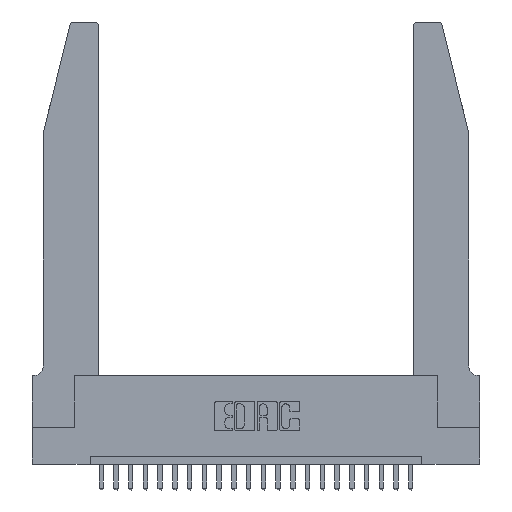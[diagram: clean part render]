
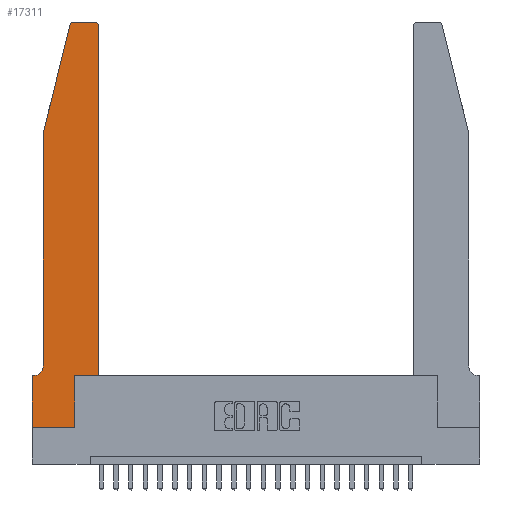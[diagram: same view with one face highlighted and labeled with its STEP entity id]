
A CAD part, top view. The second image highlights one B-rep face of the part: STEP entity #17311.
In plain terms, the highlighted planar face has unit normal (0, 0, 1).
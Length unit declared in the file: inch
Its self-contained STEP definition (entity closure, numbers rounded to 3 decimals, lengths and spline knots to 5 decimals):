
#48 = ORIENTED_EDGE ( 'NONE', *, *, #16620, .T. ) ;
#195 = ORIENTED_EDGE ( 'NONE', *, *, #9366, .T. ) ;
#345 = LINE ( 'NONE', #15022, #15609 ) ;
#792 = DIRECTION ( 'NONE',  ( -1., 0., 0. ) ) ;
#1057 = VECTOR ( 'NONE', #8726, 39.37008 ) ;
#1142 = DIRECTION ( 'NONE',  ( 1., 0., 0. ) ) ;
#1265 = CARTESIAN_POINT ( 'NONE',  ( 0., 0.35, 0.37 ) ) ;
#1666 = DIRECTION ( 'NONE',  ( 0., 0., 1. ) ) ;
#2338 = CARTESIAN_POINT ( 'NONE',  ( 0.0055, 0.35, 0.37 ) ) ;
#2448 = VERTEX_POINT ( 'NONE', #1265 ) ;
#2842 = AXIS2_PLACEMENT_3D ( 'NONE', #6579, #14122, #1142 ) ;
#3290 = LINE ( 'NONE', #15644, #8866 ) ;
#3838 = CARTESIAN_POINT ( 'NONE',  ( 0., 0., 0.37 ) ) ;
#3877 = DIRECTION ( 'NONE',  ( -1., 0., 0. ) ) ;
#4106 = AXIS2_PLACEMENT_3D ( 'NONE', #15702, #17531, #792 ) ;
#4282 = VECTOR ( 'NONE', #12554, 39.37008 ) ;
#4620 = VECTOR ( 'NONE', #15079, 39.37008 ) ;
#5086 = VERTEX_POINT ( 'NONE', #20136 ) ;
#5272 = EDGE_CURVE ( 'NONE', #6279, #13313, #17147, .T. ) ;
#5457 = CIRCLE ( 'NONE', #4106, 0.07 ) ;
#5474 = FACE_OUTER_BOUND ( 'NONE', #22347, .T. ) ;
#5493 = EDGE_CURVE ( 'NONE', #17734, #20469, #345, .T. ) ;
#5583 = CARTESIAN_POINT ( 'NONE',  ( 0.2865, 0.35, 0.37 ) ) ;
#5590 = CARTESIAN_POINT ( 'NONE',  ( 0.284, 2.75, 0.37 ) ) ;
#5680 = DIRECTION ( 'NONE',  ( -0.239, -0.971, 0. ) ) ;
#5687 = EDGE_CURVE ( 'NONE', #23686, #2448, #6239, .T. ) ;
#6239 = LINE ( 'NONE', #7975, #9727 ) ;
#6279 = VERTEX_POINT ( 'NONE', #12525 ) ;
#6579 = CARTESIAN_POINT ( 'NONE',  ( 0.4205, 2.72, 0.37 ) ) ;
#7081 = VERTEX_POINT ( 'NONE', #7574 ) ;
#7130 = CARTESIAN_POINT ( 'NONE',  ( 0., 0., 0.37 ) ) ;
#7574 = CARTESIAN_POINT ( 'NONE',  ( 0.0755, 2., 0.37 ) ) ;
#7888 = CARTESIAN_POINT ( 'NONE',  ( 0.4505, 2.72, 0.37 ) ) ;
#7975 = CARTESIAN_POINT ( 'NONE',  ( 0.0755, 0.35, 0.37 ) ) ;
#8406 = EDGE_CURVE ( 'NONE', #5086, #23686, #5457, .T. ) ;
#8726 = DIRECTION ( 'NONE',  ( 0., 1., 0. ) ) ;
#8866 = VECTOR ( 'NONE', #13930, 39.37008 ) ;
#9176 = DIRECTION ( 'NONE',  ( 1., 0., 0. ) ) ;
#9366 = EDGE_CURVE ( 'NONE', #15254, #21994, #16853, .T. ) ;
#9499 = ORIENTED_EDGE ( 'NONE', *, *, #19057, .T. ) ;
#9727 = VECTOR ( 'NONE', #13803, 39.37008 ) ;
#10662 = VERTEX_POINT ( 'NONE', #15784 ) ;
#11214 = CIRCLE ( 'NONE', #2842, 0.03 ) ;
#11333 = ORIENTED_EDGE ( 'NONE', *, *, #5687, .T. ) ;
#11573 = EDGE_CURVE ( 'NONE', #13313, #17734, #11214, .T. ) ;
#11581 = ORIENTED_EDGE ( 'NONE', *, *, #17212, .T. ) ;
#11587 = EDGE_CURVE ( 'NONE', #7081, #5086, #23654, .T. ) ;
#11641 = ORIENTED_EDGE ( 'NONE', *, *, #11573, .T. ) ;
#12249 = ORIENTED_EDGE ( 'NONE', *, *, #11587, .T. ) ;
#12305 = DIRECTION ( 'NONE',  ( 0., -1., 0. ) ) ;
#12392 = CARTESIAN_POINT ( 'NONE',  ( 0.0755, 2., 0.37 ) ) ;
#12525 = CARTESIAN_POINT ( 'NONE',  ( 0.4505, 0.35, 0.37 ) ) ;
#12552 = LINE ( 'NONE', #5583, #4620 ) ;
#12554 = DIRECTION ( 'NONE',  ( 1., 0., 0. ) ) ;
#12976 = DIRECTION ( 'NONE',  ( 1., 0., 0. ) ) ;
#13002 = CARTESIAN_POINT ( 'NONE',  ( 0.2865, 0.35, 0.37 ) ) ;
#13033 = AXIS2_PLACEMENT_3D ( 'NONE', #13135, #22411, #12976 ) ;
#13135 = CARTESIAN_POINT ( 'NONE',  ( 0., 0.35, 0.37 ) ) ;
#13313 = VERTEX_POINT ( 'NONE', #7888 ) ;
#13803 = DIRECTION ( 'NONE',  ( -1., 0., 0. ) ) ;
#13930 = DIRECTION ( 'NONE',  ( 0., -1., 0. ) ) ;
#14006 = EDGE_CURVE ( 'NONE', #20469, #10662, #17023, .T. ) ;
#14036 = VERTEX_POINT ( 'NONE', #13002 ) ;
#14122 = DIRECTION ( 'NONE',  ( 0., 0., 1. ) ) ;
#14224 = CARTESIAN_POINT ( 'NONE',  ( 0.4505, 0.35, 0.37 ) ) ;
#14437 = VECTOR ( 'NONE', #12305, 39.37008 ) ;
#14809 = CARTESIAN_POINT ( 'NONE',  ( 0.4205, 2.75, 0.37 ) ) ;
#15022 = CARTESIAN_POINT ( 'NONE',  ( 0.2605, 2.75, 0.37 ) ) ;
#15079 = DIRECTION ( 'NONE',  ( 0., 1., 0. ) ) ;
#15123 = CARTESIAN_POINT ( 'NONE',  ( 0.2865, 0., 0.37 ) ) ;
#15254 = VERTEX_POINT ( 'NONE', #3838 ) ;
#15609 = VECTOR ( 'NONE', #3877, 39.37008 ) ;
#15644 = CARTESIAN_POINT ( 'NONE',  ( 0., 0., 0.37 ) ) ;
#15686 = ORIENTED_EDGE ( 'NONE', *, *, #14006, .T. ) ;
#15702 = CARTESIAN_POINT ( 'NONE',  ( 0.0055, 0.42, 0.37 ) ) ;
#15784 = CARTESIAN_POINT ( 'NONE',  ( 0.25487, 2.72718, 0.37 ) ) ;
#16005 = LINE ( 'NONE', #19856, #4282 ) ;
#16444 = ORIENTED_EDGE ( 'NONE', *, *, #21101, .T. ) ;
#16462 = ORIENTED_EDGE ( 'NONE', *, *, #5493, .T. ) ;
#16620 = EDGE_CURVE ( 'NONE', #10662, #7081, #23847, .T. ) ;
#16853 = LINE ( 'NONE', #7130, #21216 ) ;
#17023 = CIRCLE ( 'NONE', #21631, 0.03 ) ;
#17147 = LINE ( 'NONE', #14224, #1057 ) ;
#17212 = EDGE_CURVE ( 'NONE', #21994, #14036, #12552, .T. ) ;
#17311 = ADVANCED_FACE ( 'NONE', ( #5474 ), #24020, .T. ) ;
#17531 = DIRECTION ( 'NONE',  ( 0., 0., -1. ) ) ;
#17734 = VERTEX_POINT ( 'NONE', #14809 ) ;
#18381 = VECTOR ( 'NONE', #5680, 39.37008 ) ;
#18786 = ORIENTED_EDGE ( 'NONE', *, *, #8406, .T. ) ;
#18833 = CARTESIAN_POINT ( 'NONE',  ( 0.284, 2.72, 0.37 ) ) ;
#19057 = EDGE_CURVE ( 'NONE', #14036, #6279, #16005, .T. ) ;
#19856 = CARTESIAN_POINT ( 'NONE',  ( 0.4505, 0.35, 0.37 ) ) ;
#20136 = CARTESIAN_POINT ( 'NONE',  ( 0.0755, 0.42, 0.37 ) ) ;
#20469 = VERTEX_POINT ( 'NONE', #5590 ) ;
#21101 = EDGE_CURVE ( 'NONE', #2448, #15254, #3290, .T. ) ;
#21216 = VECTOR ( 'NONE', #9176, 39.37008 ) ;
#21631 = AXIS2_PLACEMENT_3D ( 'NONE', #18833, #1666, #22205 ) ;
#21994 = VERTEX_POINT ( 'NONE', #15123 ) ;
#22123 = ORIENTED_EDGE ( 'NONE', *, *, #5272, .T. ) ;
#22205 = DIRECTION ( 'NONE',  ( 1., 0., 0. ) ) ;
#22347 = EDGE_LOOP ( 'NONE', ( #16462, #15686, #48, #12249, #18786, #11333, #16444, #195, #11581, #9499, #22123, #11641 ) ) ;
#22411 = DIRECTION ( 'NONE',  ( 0., 0., 1. ) ) ;
#23654 = LINE ( 'NONE', #12392, #14437 ) ;
#23686 = VERTEX_POINT ( 'NONE', #2338 ) ;
#23847 = LINE ( 'NONE', #24034, #18381 ) ;
#24020 = PLANE ( 'NONE',  #13033 ) ;
#24034 = CARTESIAN_POINT ( 'NONE',  ( 0.0755, 2., 0.37 ) ) ;
